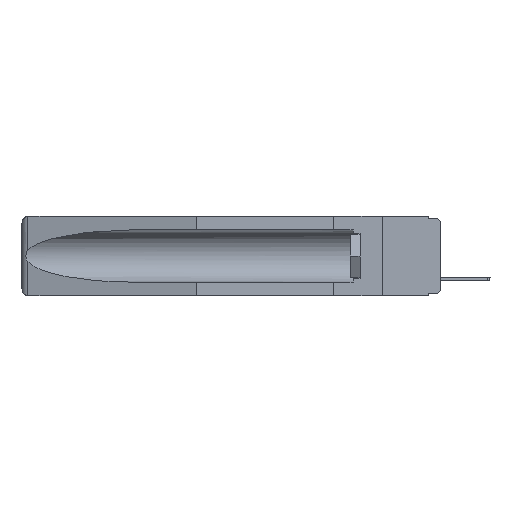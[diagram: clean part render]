
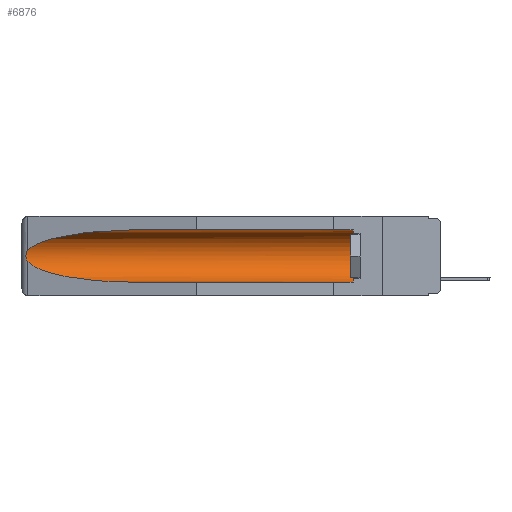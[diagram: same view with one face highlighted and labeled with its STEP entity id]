
A CAD part, left-side view. The second image highlights one B-rep face of the part: STEP entity #6876.
In plain terms, the highlighted cylindrical face has radius 2.857 mm (diameter 5.715 mm), a partial arc.
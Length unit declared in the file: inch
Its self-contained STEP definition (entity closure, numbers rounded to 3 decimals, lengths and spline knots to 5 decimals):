
#100 = VERTEX_POINT ( 'NONE', #15311 ) ;
#303 = CARTESIAN_POINT ( 'NONE',  ( 0.2673, 1.53269, -0.17917 ) ) ;
#463 = CARTESIAN_POINT ( 'NONE',  ( 0.25451, 1.48313, -0.24835 ) ) ;
#801 = CARTESIAN_POINT ( 'NONE',  ( 0.155, -0.30754, -0.1715 ) ) ;
#814 = VERTEX_POINT ( 'NONE', #14803 ) ;
#1486 = CARTESIAN_POINT ( 'NONE',  ( 0.25451, 1.48313, -0.09465 ) ) ;
#1727 = CARTESIAN_POINT ( 'NONE',  ( 0.26537, 1.52718, -0.19328 ) ) ;
#2371 = VERTEX_POINT ( 'NONE', #9196 ) ;
#2480 = CARTESIAN_POINT ( 'NONE',  ( 0.2673, 1.5327, -0.16383 ) ) ;
#2568 = DIRECTION ( 'NONE',  ( 0., 1., 0. ) ) ;
#3652 = CARTESIAN_POINT ( 'NONE',  ( 0.26654, 1.53092, -0.15636 ) ) ;
#3905 = DIRECTION ( 'NONE',  ( 0., 0., 1. ) ) ;
#4170 = EDGE_LOOP ( 'NONE', ( #9952, #7448, #10232, #13986, #6968, #8817 ) ) ;
#4224 = CARTESIAN_POINT ( 'NONE',  ( 0.21114, 1.30732, -0.284 ) ) ;
#4394 = EDGE_CURVE ( 'NONE', #2371, #13068, #8761, .T. ) ;
#4737 = DIRECTION ( 'NONE',  ( 0., 1., 0. ) ) ;
#4911 = CARTESIAN_POINT ( 'NONE',  ( 0.26537, 1.52718, -0.14972 ) ) ;
#4935 = AXIS2_PLACEMENT_3D ( 'NONE', #801, #4737, #16097 ) ;
#4955 = EDGE_CURVE ( 'NONE', #13068, #16405, #10079, .T. ) ;
#5201 = VECTOR ( 'NONE', #2568, 39.37008 ) ;
#6001 = CYLINDRICAL_SURFACE ( 'NONE', #4935, 0.1125 ) ;
#6395 = CARTESIAN_POINT ( 'NONE',  ( 0.26537, 1.52718, -0.14972 ) ) ;
#6429 = CARTESIAN_POINT ( 'NONE',  ( 0.21114, 1.30732, -0.059 ) ) ;
#6876 = ADVANCED_FACE ( 'NONE', ( #14607 ), #6001, .F. ) ;
#6968 = ORIENTED_EDGE ( 'NONE', *, *, #13915, .T. ) ;
#7030 = EDGE_CURVE ( 'NONE', #100, #2371, #12435, .T. ) ;
#7182 = EDGE_CURVE ( 'NONE', #16405, #9259, #13833, .T. ) ;
#7448 = ORIENTED_EDGE ( 'NONE', *, *, #4955, .T. ) ;
#7580 = CARTESIAN_POINT ( 'NONE',  ( 0.2675, 1.53308, -0.16763 ) ) ;
#8761 =( BOUNDED_CURVE ( )  B_SPLINE_CURVE ( 3, ( #10289, #6429, #1486, #13947 ),
 .UNSPECIFIED., .F., .T. ) 
 B_SPLINE_CURVE_WITH_KNOTS ( ( 4, 4 ),
 ( 4.71239, 6.08839 ),
 .UNSPECIFIED. ) 
 CURVE ( )  GEOMETRIC_REPRESENTATION_ITEM ( )  RATIONAL_B_SPLINE_CURVE ( ( 1., 0.848, 0.848, 1. ) ) 
 REPRESENTATION_ITEM ( '' )  );
#8817 = ORIENTED_EDGE ( 'NONE', *, *, #7030, .T. ) ;
#9196 = CARTESIAN_POINT ( 'NONE',  ( 0.155, 1.07973, -0.059 ) ) ;
#9259 = VERTEX_POINT ( 'NONE', #10630 ) ;
#9364 = CIRCLE ( 'NONE', #15194, 0.1125 ) ;
#9952 = ORIENTED_EDGE ( 'NONE', *, *, #4394, .T. ) ;
#9953 = CARTESIAN_POINT ( 'NONE',  ( 0.26597, 1.52961, -0.15275 ) ) ;
#10079 = B_SPLINE_CURVE_WITH_KNOTS ( 'NONE', 3,
 ( #4911, #9953, #3652, #2480, #7580, #12605, #303, #10357, #11763, #15752 ),
 .UNSPECIFIED., .F., .F.,
 ( 4, 2, 2, 2, 4 ),
 ( 0., 0.00029, 0.00058, 0.00087, 0.00117 ),
 .UNSPECIFIED. ) ;
#10232 = ORIENTED_EDGE ( 'NONE', *, *, #7182, .T. ) ;
#10289 = CARTESIAN_POINT ( 'NONE',  ( 0.155, 1.07973, -0.059 ) ) ;
#10357 = CARTESIAN_POINT ( 'NONE',  ( 0.26655, 1.53094, -0.18657 ) ) ;
#10630 = CARTESIAN_POINT ( 'NONE',  ( 0.155, 1.07973, -0.284 ) ) ;
#10996 = DIRECTION ( 'NONE',  ( 0., 1., 0. ) ) ;
#11526 = EDGE_CURVE ( 'NONE', #814, #9259, #16143, .T. ) ;
#11763 = CARTESIAN_POINT ( 'NONE',  ( 0.26597, 1.5296, -0.19026 ) ) ;
#12372 = VECTOR ( 'NONE', #10996, 39.37008 ) ;
#12435 = LINE ( 'NONE', #15020, #5201 ) ;
#12605 = CARTESIAN_POINT ( 'NONE',  ( 0.2675, 1.53308, -0.17534 ) ) ;
#12689 = DIRECTION ( 'NONE',  ( 0., -1., 0. ) ) ;
#12852 = CARTESIAN_POINT ( 'NONE',  ( 0.155, 1.07973, -0.284 ) ) ;
#13068 = VERTEX_POINT ( 'NONE', #6395 ) ;
#13411 = CARTESIAN_POINT ( 'NONE',  ( 0.26537, 1.52718, -0.19328 ) ) ;
#13726 = CARTESIAN_POINT ( 'NONE',  ( 0.155, -0.30754, -0.284 ) ) ;
#13833 =( BOUNDED_CURVE ( )  B_SPLINE_CURVE ( 3, ( #1727, #463, #4224, #12852 ),
 .UNSPECIFIED., .F., .T. ) 
 B_SPLINE_CURVE_WITH_KNOTS ( ( 4, 4 ),
 ( 0.1948, 1.5708 ),
 .UNSPECIFIED. ) 
 CURVE ( )  GEOMETRIC_REPRESENTATION_ITEM ( )  RATIONAL_B_SPLINE_CURVE ( ( 1., 0.848, 0.848, 1. ) ) 
 REPRESENTATION_ITEM ( '' )  );
#13915 = EDGE_CURVE ( 'NONE', #814, #100, #9364, .T. ) ;
#13936 = CARTESIAN_POINT ( 'NONE',  ( 0.155, 0.126, -0.1715 ) ) ;
#13947 = CARTESIAN_POINT ( 'NONE',  ( 0.26537, 1.52718, -0.14972 ) ) ;
#13986 = ORIENTED_EDGE ( 'NONE', *, *, #11526, .F. ) ;
#14607 = FACE_OUTER_BOUND ( 'NONE', #4170, .T. ) ;
#14803 = CARTESIAN_POINT ( 'NONE',  ( 0.155, 0.126, -0.284 ) ) ;
#15020 = CARTESIAN_POINT ( 'NONE',  ( 0.155, -0.30754, -0.059 ) ) ;
#15194 = AXIS2_PLACEMENT_3D ( 'NONE', #13936, #12689, #3905 ) ;
#15311 = CARTESIAN_POINT ( 'NONE',  ( 0.155, 0.126, -0.059 ) ) ;
#15752 = CARTESIAN_POINT ( 'NONE',  ( 0.26537, 1.52718, -0.19328 ) ) ;
#16097 = DIRECTION ( 'NONE',  ( 0., 0., 1. ) ) ;
#16143 = LINE ( 'NONE', #13726, #12372 ) ;
#16405 = VERTEX_POINT ( 'NONE', #13411 ) ;
